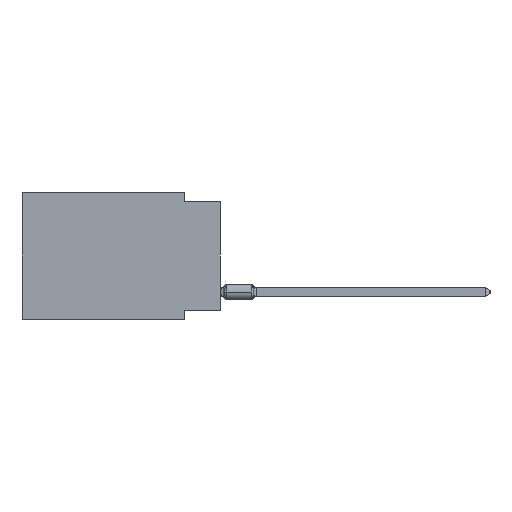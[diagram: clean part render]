
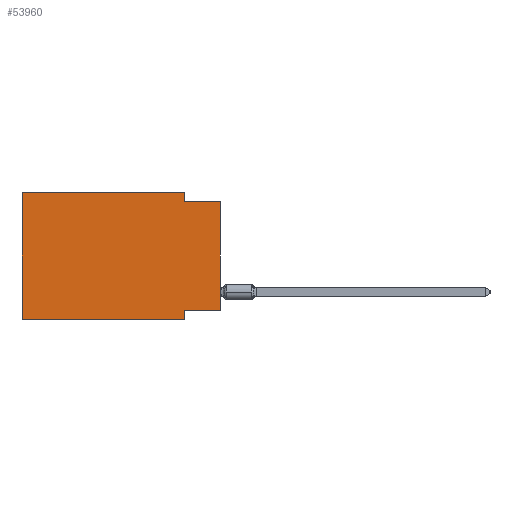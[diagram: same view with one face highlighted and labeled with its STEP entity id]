
A CAD part, left-side view. The second image highlights one B-rep face of the part: STEP entity #53960.
In plain terms, the highlighted planar face has unit normal (-1, 0, 0).
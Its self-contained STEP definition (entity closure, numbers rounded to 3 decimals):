
#1006 = DIRECTION ( 'NONE',  ( 0., 0., 1. ) ) ;
#1979 = DIRECTION ( 'NONE',  ( 0., 0., 1. ) ) ;
#2353 = VERTEX_POINT ( 'NONE', #22505 ) ;
#3785 = VECTOR ( 'NONE', #58986, 1000. ) ;
#5592 = CARTESIAN_POINT ( 'NONE',  ( 0., 13.97, 0. ) ) ;
#6191 = VECTOR ( 'NONE', #57590, 1000. ) ;
#6258 = CARTESIAN_POINT ( 'NONE',  ( 0., 2.54, -8.89 ) ) ;
#6354 = DIRECTION ( 'NONE',  ( 0., 1., 0. ) ) ;
#8631 = ORIENTED_EDGE ( 'NONE', *, *, #40718, .F. ) ;
#9320 = CARTESIAN_POINT ( 'NONE',  ( 0., 2.54, 0. ) ) ;
#11932 = CARTESIAN_POINT ( 'NONE',  ( 0., 0., -8.255 ) ) ;
#12765 = VERTEX_POINT ( 'NONE', #36718 ) ;
#15516 = EDGE_CURVE ( 'NONE', #12765, #38577, #23287, .T. ) ;
#16788 = ORIENTED_EDGE ( 'NONE', *, *, #55480, .F. ) ;
#17009 = CARTESIAN_POINT ( 'NONE',  ( 0., 2.54, -8.255 ) ) ;
#18051 = CARTESIAN_POINT ( 'NONE',  ( 0., 0., 0. ) ) ;
#20070 = PLANE ( 'NONE',  #63624 ) ;
#20203 = LINE ( 'NONE', #69123, #6191 ) ;
#21264 = CARTESIAN_POINT ( 'NONE',  ( 0., 0., -0.635 ) ) ;
#21876 = CARTESIAN_POINT ( 'NONE',  ( 0., 13.97, -8.89 ) ) ;
#22132 = ORIENTED_EDGE ( 'NONE', *, *, #61233, .F. ) ;
#22455 = VERTEX_POINT ( 'NONE', #17009 ) ;
#22505 = CARTESIAN_POINT ( 'NONE',  ( 0., 13.97, 0. ) ) ;
#23287 = LINE ( 'NONE', #18051, #43017 ) ;
#24939 = CARTESIAN_POINT ( 'NONE',  ( 0., 13.97, 0. ) ) ;
#24956 = VECTOR ( 'NONE', #1006, 1000. ) ;
#29155 = CARTESIAN_POINT ( 'NONE',  ( 0., 2.54, -0.635 ) ) ;
#33228 = ORIENTED_EDGE ( 'NONE', *, *, #15516, .T. ) ;
#36687 = CARTESIAN_POINT ( 'NONE',  ( 0., 0., -0.635 ) ) ;
#36718 = CARTESIAN_POINT ( 'NONE',  ( 0., 0., -8.255 ) ) ;
#38577 = VERTEX_POINT ( 'NONE', #36687 ) ;
#38618 = EDGE_CURVE ( 'NONE', #55561, #2353, #43320, .T. ) ;
#39874 = ORIENTED_EDGE ( 'NONE', *, *, #50346, .T. ) ;
#40075 = DIRECTION ( 'NONE',  ( 0., 0., -1. ) ) ;
#40667 = DIRECTION ( 'NONE',  ( 1., 0., 0. ) ) ;
#40718 = EDGE_CURVE ( 'NONE', #22455, #50371, #20203, .T. ) ;
#40739 = VERTEX_POINT ( 'NONE', #67734 ) ;
#41398 = ORIENTED_EDGE ( 'NONE', *, *, #64462, .F. ) ;
#43017 = VECTOR ( 'NONE', #1979, 1000. ) ;
#43320 = LINE ( 'NONE', #5592, #24956 ) ;
#43470 = EDGE_CURVE ( 'NONE', #12765, #22455, #54208, .T. ) ;
#43966 = CARTESIAN_POINT ( 'NONE',  ( 0., 13.97, -8.89 ) ) ;
#44976 = VECTOR ( 'NONE', #40075, 1000. ) ;
#45700 = VECTOR ( 'NONE', #52287, 1000. ) ;
#46627 = FACE_OUTER_BOUND ( 'NONE', #65622, .T. ) ;
#47044 = LINE ( 'NONE', #68005, #45700 ) ;
#47831 = VECTOR ( 'NONE', #6354, 1000. ) ;
#48314 = VECTOR ( 'NONE', #54799, 1000. ) ;
#50346 = EDGE_CURVE ( 'NONE', #55561, #50371, #64259, .T. ) ;
#50371 = VERTEX_POINT ( 'NONE', #6258 ) ;
#51596 = LINE ( 'NONE', #9320, #44976 ) ;
#52121 = VERTEX_POINT ( 'NONE', #29155 ) ;
#52287 = DIRECTION ( 'NONE',  ( 0., -1., 0. ) ) ;
#53960 = ADVANCED_FACE ( 'NONE', ( #46627 ), #20070, .F. ) ;
#54208 = LINE ( 'NONE', #11932, #47831 ) ;
#54799 = DIRECTION ( 'NONE',  ( 0., -1., 0. ) ) ;
#55480 = EDGE_CURVE ( 'NONE', #40739, #52121, #51596, .T. ) ;
#55561 = VERTEX_POINT ( 'NONE', #21876 ) ;
#56095 = ORIENTED_EDGE ( 'NONE', *, *, #38618, .F. ) ;
#57590 = DIRECTION ( 'NONE',  ( 0., 0., -1. ) ) ;
#57801 = DIRECTION ( 'NONE',  ( 0., 0., -1. ) ) ;
#58986 = DIRECTION ( 'NONE',  ( 0., -1., 0. ) ) ;
#59196 = ORIENTED_EDGE ( 'NONE', *, *, #43470, .F. ) ;
#61233 = EDGE_CURVE ( 'NONE', #52121, #38577, #63544, .T. ) ;
#63544 = LINE ( 'NONE', #21264, #3785 ) ;
#63624 = AXIS2_PLACEMENT_3D ( 'NONE', #24939, #40667, #57801 ) ;
#64259 = LINE ( 'NONE', #43966, #48314 ) ;
#64462 = EDGE_CURVE ( 'NONE', #2353, #40739, #47044, .T. ) ;
#65622 = EDGE_LOOP ( 'NONE', ( #33228, #22132, #16788, #41398, #56095, #39874, #8631, #59196 ) ) ;
#67734 = CARTESIAN_POINT ( 'NONE',  ( 0., 2.54, 0. ) ) ;
#68005 = CARTESIAN_POINT ( 'NONE',  ( 0., 13.97, 0. ) ) ;
#69123 = CARTESIAN_POINT ( 'NONE',  ( 0., 2.54, -8.89 ) ) ;
